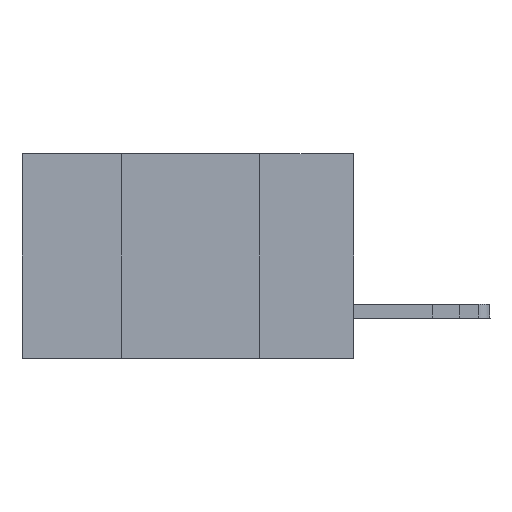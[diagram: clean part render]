
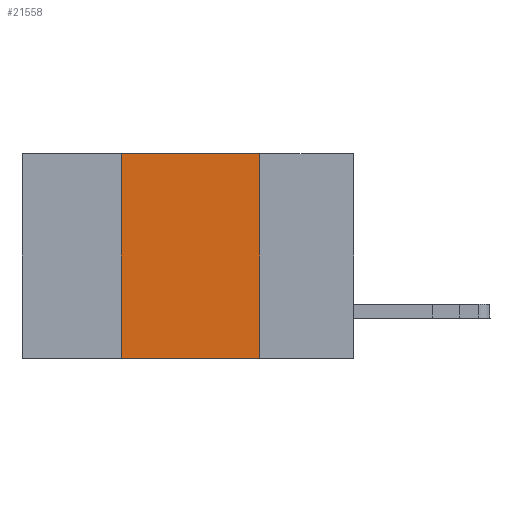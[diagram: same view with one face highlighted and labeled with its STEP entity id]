
A CAD part, left-side view. The second image highlights one B-rep face of the part: STEP entity #21558.
In plain terms, the highlighted planar face has unit normal (-1, 0, 0).
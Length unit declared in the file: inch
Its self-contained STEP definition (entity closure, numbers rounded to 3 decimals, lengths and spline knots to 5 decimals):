
#314 = VERTEX_POINT ( 'NONE', #12907 ) ;
#897 = EDGE_CURVE ( 'NONE', #314, #20508, #16997, .T. ) ;
#1505 = EDGE_CURVE ( 'NONE', #4810, #314, #13461, .T. ) ;
#1854 = CARTESIAN_POINT ( 'NONE',  ( 0., 0.17, 0. ) ) ;
#2784 = VECTOR ( 'NONE', #18928, 39.37008 ) ;
#3458 = LINE ( 'NONE', #4948, #17894 ) ;
#4810 = VERTEX_POINT ( 'NONE', #22063 ) ;
#4873 = DIRECTION ( 'NONE',  ( 0., -1., 0. ) ) ;
#4948 = CARTESIAN_POINT ( 'NONE',  ( 0., 0.6, -0.37 ) ) ;
#5112 = VECTOR ( 'NONE', #13221, 39.37008 ) ;
#6630 = DIRECTION ( 'NONE',  ( 1., 0., 0. ) ) ;
#6736 = EDGE_CURVE ( 'NONE', #4810, #19869, #3458, .T. ) ;
#7065 = VECTOR ( 'NONE', #12575, 39.37008 ) ;
#7141 = CARTESIAN_POINT ( 'NONE',  ( 0., 0.17, -0.37 ) ) ;
#8478 = CARTESIAN_POINT ( 'NONE',  ( 0., 0.42, 0. ) ) ;
#10963 = CARTESIAN_POINT ( 'NONE',  ( 0., 0.17, 0. ) ) ;
#11081 = AXIS2_PLACEMENT_3D ( 'NONE', #17801, #6630, #19657 ) ;
#12208 = PLANE ( 'NONE',  #11081 ) ;
#12575 = DIRECTION ( 'NONE',  ( 0., -1., 0. ) ) ;
#12583 = ORIENTED_EDGE ( 'NONE', *, *, #19041, .F. ) ;
#12907 = CARTESIAN_POINT ( 'NONE',  ( 0., 0.42, 0. ) ) ;
#13221 = DIRECTION ( 'NONE',  ( 0., 0., -1. ) ) ;
#13461 = LINE ( 'NONE', #8478, #2784 ) ;
#13564 = CARTESIAN_POINT ( 'NONE',  ( 0., 0.6, 0. ) ) ;
#13632 = ORIENTED_EDGE ( 'NONE', *, *, #897, .F. ) ;
#15161 = LINE ( 'NONE', #1854, #5112 ) ;
#15222 = ORIENTED_EDGE ( 'NONE', *, *, #1505, .F. ) ;
#16997 = LINE ( 'NONE', #13564, #7065 ) ;
#17801 = CARTESIAN_POINT ( 'NONE',  ( 0., 0.6, 0. ) ) ;
#17894 = VECTOR ( 'NONE', #4873, 39.37008 ) ;
#18928 = DIRECTION ( 'NONE',  ( 0., 0., 1. ) ) ;
#19041 = EDGE_CURVE ( 'NONE', #20508, #19869, #15161, .T. ) ;
#19374 = FACE_OUTER_BOUND ( 'NONE', #21647, .T. ) ;
#19657 = DIRECTION ( 'NONE',  ( 0., 0., -1. ) ) ;
#19869 = VERTEX_POINT ( 'NONE', #7141 ) ;
#20508 = VERTEX_POINT ( 'NONE', #10963 ) ;
#20919 = ORIENTED_EDGE ( 'NONE', *, *, #6736, .T. ) ;
#21558 = ADVANCED_FACE ( 'NONE', ( #19374 ), #12208, .F. ) ;
#21647 = EDGE_LOOP ( 'NONE', ( #12583, #13632, #15222, #20919 ) ) ;
#22063 = CARTESIAN_POINT ( 'NONE',  ( 0., 0.42, -0.37 ) ) ;
